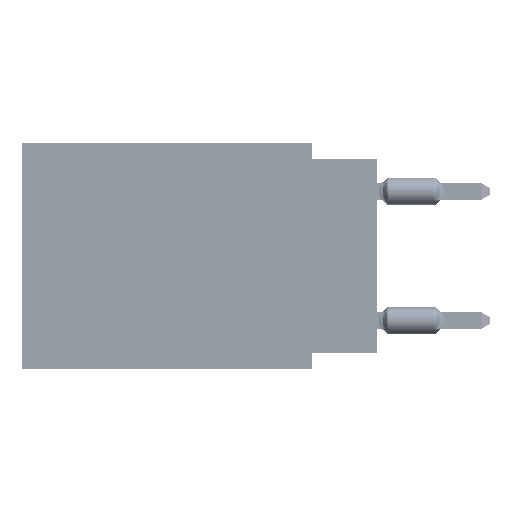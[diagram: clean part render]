
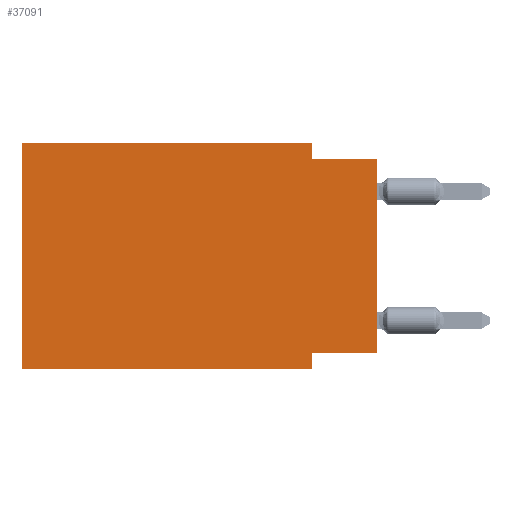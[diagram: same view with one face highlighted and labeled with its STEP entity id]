
A CAD part, left-side view. The second image highlights one B-rep face of the part: STEP entity #37091.
In plain terms, the highlighted planar face has unit normal (-1, 0, 0).
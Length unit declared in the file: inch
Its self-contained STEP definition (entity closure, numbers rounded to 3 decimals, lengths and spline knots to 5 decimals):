
#224 = EDGE_CURVE ( 'NONE', #4923, #77977, #12469, .T. ) ;
#1670 = ORIENTED_EDGE ( 'NONE', *, *, #61786, .F. ) ;
#2472 = EDGE_CURVE ( 'NONE', #32374, #14305, #43600, .T. ) ;
#3379 = CARTESIAN_POINT ( 'NONE',  ( 0., 0., -0.025 ) ) ;
#3778 = DIRECTION ( 'NONE',  ( 0., 0., -1. ) ) ;
#4084 = VECTOR ( 'NONE', #13188, 39.37008 ) ;
#4809 = ORIENTED_EDGE ( 'NONE', *, *, #36145, .F. ) ;
#4923 = VERTEX_POINT ( 'NONE', #17157 ) ;
#6689 = VERTEX_POINT ( 'NONE', #59037 ) ;
#7010 = ORIENTED_EDGE ( 'NONE', *, *, #224, .F. ) ;
#7706 = EDGE_CURVE ( 'NONE', #77977, #45831, #42033, .T. ) ;
#8803 = CARTESIAN_POINT ( 'NONE',  ( 0., 0.1, -0.025 ) ) ;
#9124 = LINE ( 'NONE', #67105, #40533 ) ;
#9157 = DIRECTION ( 'NONE',  ( 1., 0., 0. ) ) ;
#9578 = CARTESIAN_POINT ( 'NONE',  ( 0., 0., -0.325 ) ) ;
#12469 = LINE ( 'NONE', #65758, #58667 ) ;
#13188 = DIRECTION ( 'NONE',  ( 0., 0., -1. ) ) ;
#14305 = VERTEX_POINT ( 'NONE', #73888 ) ;
#15559 = LINE ( 'NONE', #71986, #30348 ) ;
#15889 = DIRECTION ( 'NONE',  ( 0., 1., 0. ) ) ;
#16552 = DIRECTION ( 'NONE',  ( 0., 0., 1. ) ) ;
#17157 = CARTESIAN_POINT ( 'NONE',  ( 0., 0.55, -0.35 ) ) ;
#20710 = DIRECTION ( 'NONE',  ( 0., -1., 0. ) ) ;
#22401 = CARTESIAN_POINT ( 'NONE',  ( 0., 0.55, 0. ) ) ;
#23354 = VECTOR ( 'NONE', #15889, 39.37008 ) ;
#24672 = VERTEX_POINT ( 'NONE', #8803 ) ;
#25015 = ORIENTED_EDGE ( 'NONE', *, *, #69940, .T. ) ;
#28035 = DIRECTION ( 'NONE',  ( 0., -1., 0. ) ) ;
#28056 = FACE_OUTER_BOUND ( 'NONE', #42777, .T. ) ;
#28727 = ORIENTED_EDGE ( 'NONE', *, *, #7706, .F. ) ;
#30348 = VECTOR ( 'NONE', #28035, 39.37008 ) ;
#32374 = VERTEX_POINT ( 'NONE', #46308 ) ;
#36145 = EDGE_CURVE ( 'NONE', #6689, #32374, #39978, .T. ) ;
#37091 = ADVANCED_FACE ( 'NONE', ( #28056 ), #71827, .F. ) ;
#39978 = LINE ( 'NONE', #9578, #23354 ) ;
#40533 = VECTOR ( 'NONE', #16552, 39.37008 ) ;
#42033 = LINE ( 'NONE', #64394, #73557 ) ;
#42488 = LINE ( 'NONE', #76187, #73997 ) ;
#42777 = EDGE_LOOP ( 'NONE', ( #51552, #74283, #1670, #28727, #7010, #25015, #42993, #4809 ) ) ;
#42993 = ORIENTED_EDGE ( 'NONE', *, *, #2472, .F. ) ;
#43600 = LINE ( 'NONE', #54034, #56401 ) ;
#44746 = CARTESIAN_POINT ( 'NONE',  ( 0., 0.1, 0. ) ) ;
#45831 = VERTEX_POINT ( 'NONE', #63645 ) ;
#46308 = CARTESIAN_POINT ( 'NONE',  ( 0., 0.1, -0.325 ) ) ;
#46780 = CARTESIAN_POINT ( 'NONE',  ( 0., 0.55, 0. ) ) ;
#51100 = VERTEX_POINT ( 'NONE', #3379 ) ;
#51552 = ORIENTED_EDGE ( 'NONE', *, *, #61082, .T. ) ;
#53082 = DIRECTION ( 'NONE',  ( 0., 0., 1. ) ) ;
#53088 = DIRECTION ( 'NONE',  ( 0., 0., -1. ) ) ;
#53366 = AXIS2_PLACEMENT_3D ( 'NONE', #46780, #9157, #53088 ) ;
#54034 = CARTESIAN_POINT ( 'NONE',  ( 0., 0.1, -0.35 ) ) ;
#54219 = LINE ( 'NONE', #44746, #4084 ) ;
#56401 = VECTOR ( 'NONE', #3778, 39.37008 ) ;
#57466 = DIRECTION ( 'NONE',  ( 0., -1., 0. ) ) ;
#58667 = VECTOR ( 'NONE', #53082, 39.37008 ) ;
#59037 = CARTESIAN_POINT ( 'NONE',  ( 0., 0., -0.325 ) ) ;
#61082 = EDGE_CURVE ( 'NONE', #6689, #51100, #9124, .T. ) ;
#61786 = EDGE_CURVE ( 'NONE', #45831, #24672, #54219, .T. ) ;
#63645 = CARTESIAN_POINT ( 'NONE',  ( 0., 0.1, 0. ) ) ;
#64394 = CARTESIAN_POINT ( 'NONE',  ( 0., 0.55, 0. ) ) ;
#65758 = CARTESIAN_POINT ( 'NONE',  ( 0., 0.55, 0. ) ) ;
#67105 = CARTESIAN_POINT ( 'NONE',  ( 0., 0., 0. ) ) ;
#69940 = EDGE_CURVE ( 'NONE', #4923, #14305, #42488, .T. ) ;
#71827 = PLANE ( 'NONE',  #53366 ) ;
#71986 = CARTESIAN_POINT ( 'NONE',  ( 0., 0., -0.025 ) ) ;
#73557 = VECTOR ( 'NONE', #20710, 39.37008 ) ;
#73888 = CARTESIAN_POINT ( 'NONE',  ( 0., 0.1, -0.35 ) ) ;
#73997 = VECTOR ( 'NONE', #57466, 39.37008 ) ;
#74283 = ORIENTED_EDGE ( 'NONE', *, *, #79150, .F. ) ;
#76187 = CARTESIAN_POINT ( 'NONE',  ( 0., 0.55, -0.35 ) ) ;
#77977 = VERTEX_POINT ( 'NONE', #22401 ) ;
#79150 = EDGE_CURVE ( 'NONE', #24672, #51100, #15559, .T. ) ;
